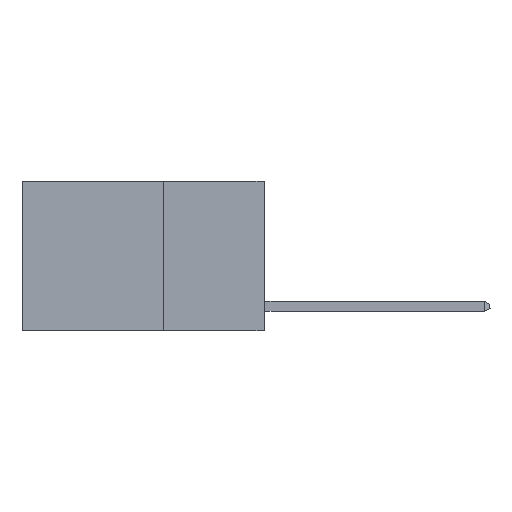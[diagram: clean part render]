
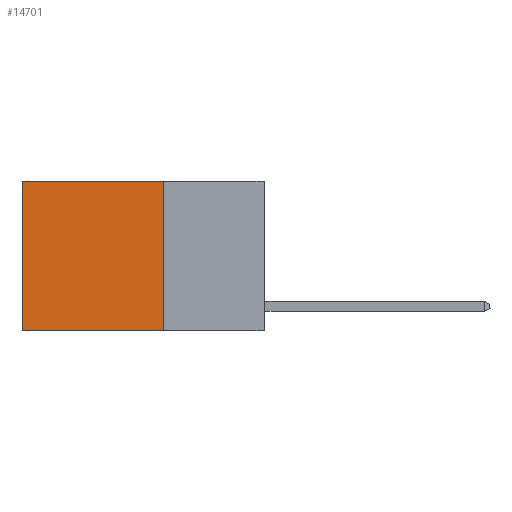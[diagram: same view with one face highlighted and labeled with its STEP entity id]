
A CAD part, left-side view. The second image highlights one B-rep face of the part: STEP entity #14701.
In plain terms, the highlighted planar face has unit normal (-1, 0, 0).
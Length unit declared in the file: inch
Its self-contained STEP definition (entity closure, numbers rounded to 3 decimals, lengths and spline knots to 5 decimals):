
#40 = FACE_OUTER_BOUND ( 'NONE', #2508, .T. ) ;
#141 = ORIENTED_EDGE ( 'NONE', *, *, #11595, .T. ) ;
#1001 = CARTESIAN_POINT ( 'NONE',  ( 0.2625, 0.6, -0.37 ) ) ;
#1616 = DIRECTION ( 'NONE',  ( 0., 1., 0. ) ) ;
#2401 = ORIENTED_EDGE ( 'NONE', *, *, #12324, .F. ) ;
#2410 = LINE ( 'NONE', #6991, #8106 ) ;
#2428 = VERTEX_POINT ( 'NONE', #4675 ) ;
#2508 = EDGE_LOOP ( 'NONE', ( #141, #2401, #11214, #12613 ) ) ;
#2777 = LINE ( 'NONE', #7332, #5499 ) ;
#4039 = VECTOR ( 'NONE', #4504, 39.37008 ) ;
#4504 = DIRECTION ( 'NONE',  ( 0., 0., -1. ) ) ;
#4647 = CARTESIAN_POINT ( 'NONE',  ( 0.2625, 0.6, 0. ) ) ;
#4675 = CARTESIAN_POINT ( 'NONE',  ( 0.2625, 0.25, -0.37 ) ) ;
#5499 = VECTOR ( 'NONE', #1616, 39.37008 ) ;
#6565 = LINE ( 'NONE', #11022, #12664 ) ;
#6991 = CARTESIAN_POINT ( 'NONE',  ( 0.2625, 0.25, 0. ) ) ;
#7332 = CARTESIAN_POINT ( 'NONE',  ( 0.2625, 0.25, -0.37 ) ) ;
#7839 = VERTEX_POINT ( 'NONE', #9019 ) ;
#8106 = VECTOR ( 'NONE', #11604, 39.37008 ) ;
#9019 = CARTESIAN_POINT ( 'NONE',  ( 0.2625, 0.6, 0. ) ) ;
#9314 = DIRECTION ( 'NONE',  ( 1., 0., 0. ) ) ;
#9397 = AXIS2_PLACEMENT_3D ( 'NONE', #14717, #9314, #10432 ) ;
#10153 = LINE ( 'NONE', #4647, #4039 ) ;
#10432 = DIRECTION ( 'NONE',  ( 0., 0., -1. ) ) ;
#10597 = VERTEX_POINT ( 'NONE', #1001 ) ;
#11012 = EDGE_CURVE ( 'NONE', #12800, #2428, #6565, .T. ) ;
#11022 = CARTESIAN_POINT ( 'NONE',  ( 0.2625, 0.25, 0. ) ) ;
#11214 = ORIENTED_EDGE ( 'NONE', *, *, #11012, .F. ) ;
#11595 = EDGE_CURVE ( 'NONE', #7839, #10597, #10153, .T. ) ;
#11599 = EDGE_CURVE ( 'NONE', #12800, #7839, #2410, .T. ) ;
#11604 = DIRECTION ( 'NONE',  ( 0., 1., 0. ) ) ;
#12324 = EDGE_CURVE ( 'NONE', #2428, #10597, #2777, .T. ) ;
#12499 = CARTESIAN_POINT ( 'NONE',  ( 0.2625, 0.25, 0. ) ) ;
#12613 = ORIENTED_EDGE ( 'NONE', *, *, #11599, .T. ) ;
#12664 = VECTOR ( 'NONE', #13275, 39.37008 ) ;
#12800 = VERTEX_POINT ( 'NONE', #12499 ) ;
#13275 = DIRECTION ( 'NONE',  ( 0., 0., -1. ) ) ;
#13921 = PLANE ( 'NONE',  #9397 ) ;
#14701 = ADVANCED_FACE ( 'NONE', ( #40 ), #13921, .F. ) ;
#14717 = CARTESIAN_POINT ( 'NONE',  ( 0.2625, 0.25, 0. ) ) ;
